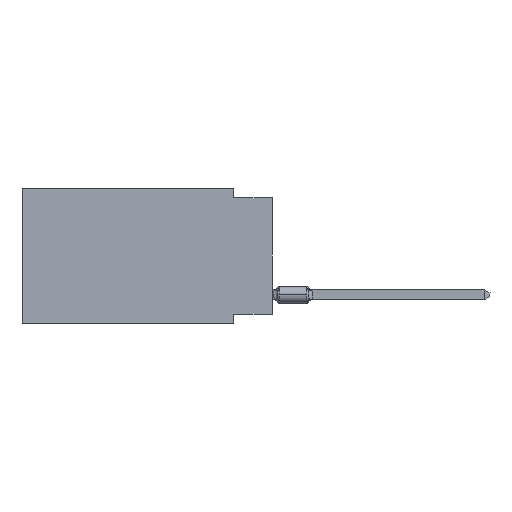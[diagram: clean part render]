
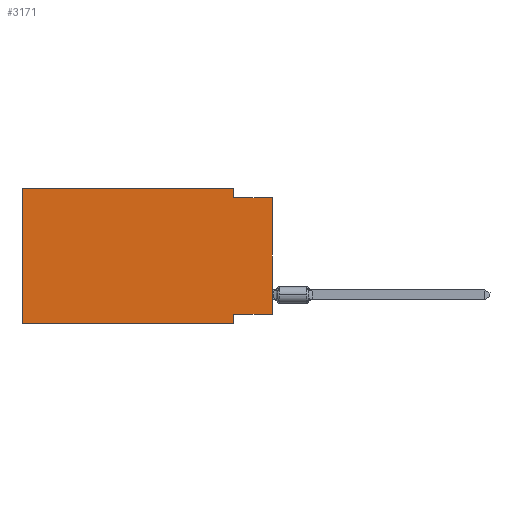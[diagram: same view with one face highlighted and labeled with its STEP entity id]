
A CAD part, left-side view. The second image highlights one B-rep face of the part: STEP entity #3171.
In plain terms, the highlighted planar face has unit normal (-1, 0, 0).
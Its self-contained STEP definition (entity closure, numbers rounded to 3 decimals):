
#40 = DIRECTION ( 'NONE',  ( 0., -1., 0. ) ) ;
#1094 = VERTEX_POINT ( 'NONE', #9540 ) ;
#1177 = CARTESIAN_POINT ( 'NONE',  ( 0., 2.54, -0.635 ) ) ;
#1313 = CARTESIAN_POINT ( 'NONE',  ( 0., 16.383, 0. ) ) ;
#1557 = VECTOR ( 'NONE', #12329, 1000. ) ;
#2062 = CARTESIAN_POINT ( 'NONE',  ( 0., 2.54, -8.89 ) ) ;
#2105 = ORIENTED_EDGE ( 'NONE', *, *, #10765, .F. ) ;
#2154 = ORIENTED_EDGE ( 'NONE', *, *, #4028, .F. ) ;
#2158 = LINE ( 'NONE', #2062, #13694 ) ;
#2179 = DIRECTION ( 'NONE',  ( 0., 0., -1. ) ) ;
#2747 = CARTESIAN_POINT ( 'NONE',  ( 0., 0., -8.255 ) ) ;
#3167 = DIRECTION ( 'NONE',  ( 0., 0., 1. ) ) ;
#3171 = ADVANCED_FACE ( 'NONE', ( #18603 ), #9502, .F. ) ;
#4028 = EDGE_CURVE ( 'NONE', #16873, #16955, #8270, .T. ) ;
#4145 = ORIENTED_EDGE ( 'NONE', *, *, #13044, .T. ) ;
#4549 = LINE ( 'NONE', #7973, #5417 ) ;
#4668 = VECTOR ( 'NONE', #5388, 1000. ) ;
#4774 = CARTESIAN_POINT ( 'NONE',  ( 0., 0., 0. ) ) ;
#4894 = EDGE_CURVE ( 'NONE', #7998, #4920, #7937, .T. ) ;
#4920 = VERTEX_POINT ( 'NONE', #17775 ) ;
#4927 = EDGE_LOOP ( 'NONE', ( #4145, #13236, #2154, #13906, #17810, #8415, #2105, #5686 ) ) ;
#4930 = CARTESIAN_POINT ( 'NONE',  ( 0., 2.54, 0. ) ) ;
#5388 = DIRECTION ( 'NONE',  ( 0., -1., 0. ) ) ;
#5417 = VECTOR ( 'NONE', #3167, 1000. ) ;
#5686 = ORIENTED_EDGE ( 'NONE', *, *, #4894, .F. ) ;
#5892 = CARTESIAN_POINT ( 'NONE',  ( 0., 2.54, -8.89 ) ) ;
#6269 = VECTOR ( 'NONE', #40, 1000. ) ;
#6795 = DIRECTION ( 'NONE',  ( 0., -1., 0. ) ) ;
#6901 = LINE ( 'NONE', #10135, #10935 ) ;
#7653 = EDGE_CURVE ( 'NONE', #11827, #11747, #4549, .T. ) ;
#7932 = DIRECTION ( 'NONE',  ( 0., 0., -1. ) ) ;
#7937 = LINE ( 'NONE', #17135, #10484 ) ;
#7973 = CARTESIAN_POINT ( 'NONE',  ( 0., 16.383, 0. ) ) ;
#7998 = VERTEX_POINT ( 'NONE', #2747 ) ;
#8270 = LINE ( 'NONE', #17286, #11295 ) ;
#8415 = ORIENTED_EDGE ( 'NONE', *, *, #14005, .T. ) ;
#8679 = CARTESIAN_POINT ( 'NONE',  ( 0., 16.383, 0. ) ) ;
#9502 = PLANE ( 'NONE',  #15643 ) ;
#9540 = CARTESIAN_POINT ( 'NONE',  ( 0., 0., -0.635 ) ) ;
#9597 = DIRECTION ( 'NONE',  ( 1., 0., 0. ) ) ;
#9810 = LINE ( 'NONE', #15786, #4668 ) ;
#10135 = CARTESIAN_POINT ( 'NONE',  ( 0., 0., -0.635 ) ) ;
#10484 = VECTOR ( 'NONE', #12634, 1000. ) ;
#10765 = EDGE_CURVE ( 'NONE', #4920, #18221, #2158, .T. ) ;
#10935 = VECTOR ( 'NONE', #6795, 1000. ) ;
#11075 = CARTESIAN_POINT ( 'NONE',  ( 0., 16.383, 0. ) ) ;
#11295 = VECTOR ( 'NONE', #2179, 1000. ) ;
#11747 = VERTEX_POINT ( 'NONE', #1313 ) ;
#11827 = VERTEX_POINT ( 'NONE', #13370 ) ;
#12155 = EDGE_CURVE ( 'NONE', #16955, #1094, #6901, .T. ) ;
#12329 = DIRECTION ( 'NONE',  ( 0., 0., 1. ) ) ;
#12634 = DIRECTION ( 'NONE',  ( 0., 1., 0. ) ) ;
#13044 = EDGE_CURVE ( 'NONE', #7998, #1094, #13890, .T. ) ;
#13236 = ORIENTED_EDGE ( 'NONE', *, *, #12155, .F. ) ;
#13370 = CARTESIAN_POINT ( 'NONE',  ( 0., 16.383, -8.89 ) ) ;
#13694 = VECTOR ( 'NONE', #16974, 1000. ) ;
#13890 = LINE ( 'NONE', #4774, #1557 ) ;
#13906 = ORIENTED_EDGE ( 'NONE', *, *, #14525, .F. ) ;
#14005 = EDGE_CURVE ( 'NONE', #11827, #18221, #9810, .T. ) ;
#14525 = EDGE_CURVE ( 'NONE', #11747, #16873, #16336, .T. ) ;
#15643 = AXIS2_PLACEMENT_3D ( 'NONE', #11075, #9597, #7932 ) ;
#15786 = CARTESIAN_POINT ( 'NONE',  ( 0., 16.383, -8.89 ) ) ;
#16336 = LINE ( 'NONE', #8679, #6269 ) ;
#16873 = VERTEX_POINT ( 'NONE', #4930 ) ;
#16955 = VERTEX_POINT ( 'NONE', #1177 ) ;
#16974 = DIRECTION ( 'NONE',  ( 0., 0., -1. ) ) ;
#17135 = CARTESIAN_POINT ( 'NONE',  ( 0., 0., -8.255 ) ) ;
#17286 = CARTESIAN_POINT ( 'NONE',  ( 0., 2.54, 0. ) ) ;
#17775 = CARTESIAN_POINT ( 'NONE',  ( 0., 2.54, -8.255 ) ) ;
#17810 = ORIENTED_EDGE ( 'NONE', *, *, #7653, .F. ) ;
#18221 = VERTEX_POINT ( 'NONE', #5892 ) ;
#18603 = FACE_OUTER_BOUND ( 'NONE', #4927, .T. ) ;
